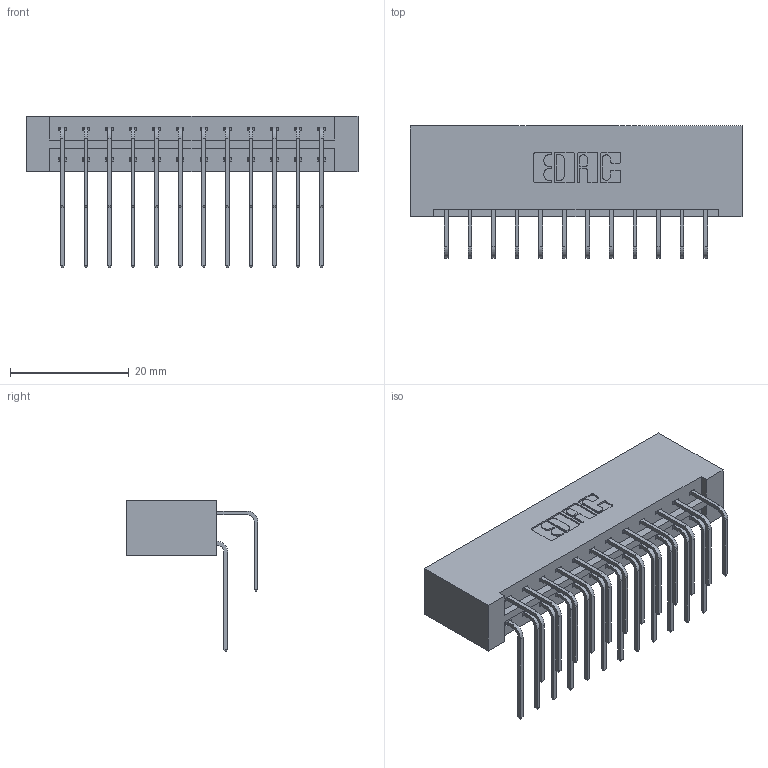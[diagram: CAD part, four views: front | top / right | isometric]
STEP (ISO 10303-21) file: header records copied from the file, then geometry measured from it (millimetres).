
FILE_DESCRIPTION (( 'STEP AP203' ), '1' );
FILE_NAME ('333-024-558-201.STEP', '2018-08-02T11:39:19', ( '' ), ( '' ), 'SwSTEP 2.0', 'SolidWorks 2016', '' );
FILE_SCHEMA (( 'CONFIG_CONTROL_DESIGN' ));
Length unit declared in the file: inch
Products named in the file (4): 345-292-001_558 Tail - 2; 333 Part_Lugless; 333-024-558-201; 345-292-001_558 559 Tail - 1
Assembly tree (25 placements, depth 2):
  333-024-558-201
    333 Part_Lugless
    345-292-001_558 559 Tail - 1  x12
    345-292-001_558 Tail - 2  x12
Bounding box: 55.8 x 22.17 x 25.53 mm (x, y, z)
Volume: 6187.4 mm3; surface area: 7706.6 mm2
Topology: 25 solids, 25 shells, 1402 faces, 4151 edges, 2734 vertices
Faces by surface type: plane 978, cylinder 424
Entity records: 13107 total; most frequent: CARTESIAN_POINT 2257, ORIENTED_EDGE 2142, DIRECTION 1955, EDGE_CURVE 1071, VECTOR 911, LINE 911, VERTEX_POINT 710, AXIS2_PLACEMENT_3D 522
